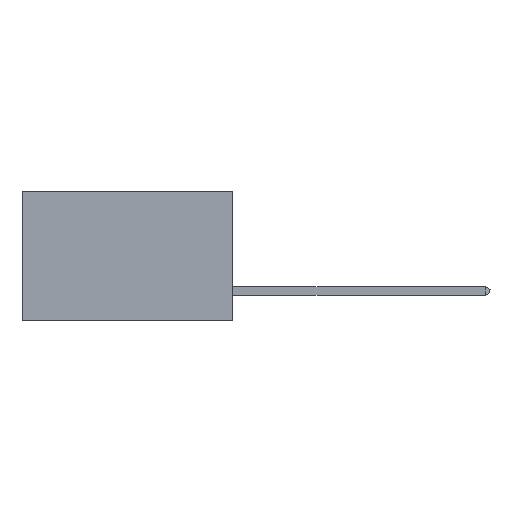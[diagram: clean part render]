
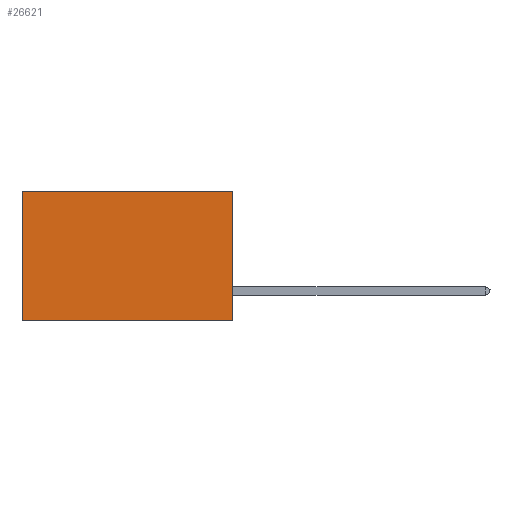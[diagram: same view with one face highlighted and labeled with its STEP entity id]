
A CAD part, left-side view. The second image highlights one B-rep face of the part: STEP entity #26621.
In plain terms, the highlighted planar face has unit normal (-1, 0, 0).
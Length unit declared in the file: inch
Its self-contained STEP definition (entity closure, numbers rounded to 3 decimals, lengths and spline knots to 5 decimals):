
#354 = ORIENTED_EDGE ( 'NONE', *, *, #9217, .T. ) ;
#1806 = CARTESIAN_POINT ( 'NONE',  ( 0.2875, 0.6, -0.37 ) ) ;
#1841 = LINE ( 'NONE', #6102, #17111 ) ;
#2794 = CARTESIAN_POINT ( 'NONE',  ( 0.2875, 0.6, 0. ) ) ;
#2860 = VERTEX_POINT ( 'NONE', #4671 ) ;
#4482 = EDGE_LOOP ( 'NONE', ( #354, #6542, #17727, #15253 ) ) ;
#4671 = CARTESIAN_POINT ( 'NONE',  ( 0.2875, 0.6, 0. ) ) ;
#6102 = CARTESIAN_POINT ( 'NONE',  ( 0.2875, 0., 0. ) ) ;
#6542 = ORIENTED_EDGE ( 'NONE', *, *, #8261, .F. ) ;
#7459 = CARTESIAN_POINT ( 'NONE',  ( 0.2875, 0., -0.37 ) ) ;
#7732 = CARTESIAN_POINT ( 'NONE',  ( 0.2875, 0., 0. ) ) ;
#8111 = VERTEX_POINT ( 'NONE', #7459 ) ;
#8261 = EDGE_CURVE ( 'NONE', #8111, #21370, #12331, .T. ) ;
#9217 = EDGE_CURVE ( 'NONE', #2860, #21370, #12946, .T. ) ;
#9805 = AXIS2_PLACEMENT_3D ( 'NONE', #23913, #21734, #12619 ) ;
#10424 = PLANE ( 'NONE',  #9805 ) ;
#10563 = VECTOR ( 'NONE', #21567, 39.37008 ) ;
#12331 = LINE ( 'NONE', #14966, #10563 ) ;
#12619 = DIRECTION ( 'NONE',  ( 0., 0., -1. ) ) ;
#12946 = LINE ( 'NONE', #2794, #22624 ) ;
#13892 = VECTOR ( 'NONE', #25876, 39.37008 ) ;
#14966 = CARTESIAN_POINT ( 'NONE',  ( 0.2875, 0., -0.37 ) ) ;
#15089 = CARTESIAN_POINT ( 'NONE',  ( 0.2875, 0., 0. ) ) ;
#15253 = ORIENTED_EDGE ( 'NONE', *, *, #21451, .T. ) ;
#17111 = VECTOR ( 'NONE', #19936, 39.37008 ) ;
#17727 = ORIENTED_EDGE ( 'NONE', *, *, #20776, .F. ) ;
#18690 = DIRECTION ( 'NONE',  ( 0., 0., -1. ) ) ;
#19936 = DIRECTION ( 'NONE',  ( 0., 1., 0. ) ) ;
#20776 = EDGE_CURVE ( 'NONE', #21964, #8111, #23589, .T. ) ;
#21370 = VERTEX_POINT ( 'NONE', #1806 ) ;
#21451 = EDGE_CURVE ( 'NONE', #21964, #2860, #1841, .T. ) ;
#21567 = DIRECTION ( 'NONE',  ( 0., 1., 0. ) ) ;
#21734 = DIRECTION ( 'NONE',  ( 1., 0., 0. ) ) ;
#21964 = VERTEX_POINT ( 'NONE', #15089 ) ;
#22624 = VECTOR ( 'NONE', #18690, 39.37008 ) ;
#23589 = LINE ( 'NONE', #7732, #13892 ) ;
#23913 = CARTESIAN_POINT ( 'NONE',  ( 0.2875, 0., 0. ) ) ;
#25876 = DIRECTION ( 'NONE',  ( 0., 0., -1. ) ) ;
#26621 = ADVANCED_FACE ( 'NONE', ( #29044 ), #10424, .F. ) ;
#29044 = FACE_OUTER_BOUND ( 'NONE', #4482, .T. ) ;
